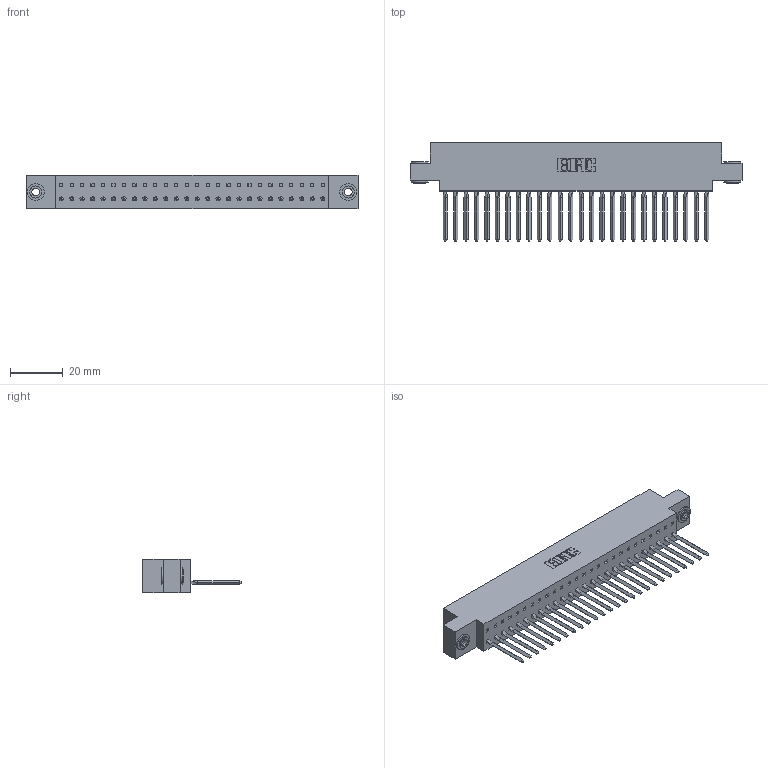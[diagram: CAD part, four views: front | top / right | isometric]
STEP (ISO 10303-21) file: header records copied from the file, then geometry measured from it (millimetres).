
FILE_DESCRIPTION (( 'STEP AP203' ), '1' );
FILE_NAME ('317-026-541-603.STEP', '2020-02-27T18:42:30', ( '' ), ( '' ), 'SwSTEP 2.0', 'SolidWorks 2016', '' );
FILE_SCHEMA (( 'CONFIG_CONTROL_DESIGN' ));
Length unit declared in the file: inch
Products named in the file (4): 317-290-002_541; 345-250-002_345-250-002-102; 317-026-541-603; 317 Part_.156 Dia - TH
Assembly tree (29 placements, depth 2):
  317-026-541-603
    317 Part_.156 Dia - TH
    317-290-002_541  x26
    345-250-002_345-250-002-102  x2
Bounding box: 125.73 x 37.34 x 12.7 mm (x, y, z)
Volume: 19916.6 mm3; surface area: 27824.7 mm2
Topology: 29 solids, 29 shells, 4092 faces, 11635 edges, 7562 vertices
Faces by surface type: plane 3292, cylinder 688, bspline 104, cone 8
Entity records: 41181 total; most frequent: CARTESIAN_POINT 7922, ORIENTED_EDGE 7194, DIRECTION 5939, EDGE_CURVE 3597, VECTOR 3209, LINE 3209, VERTEX_POINT 2388, AXIS2_PLACEMENT_3D 1365
